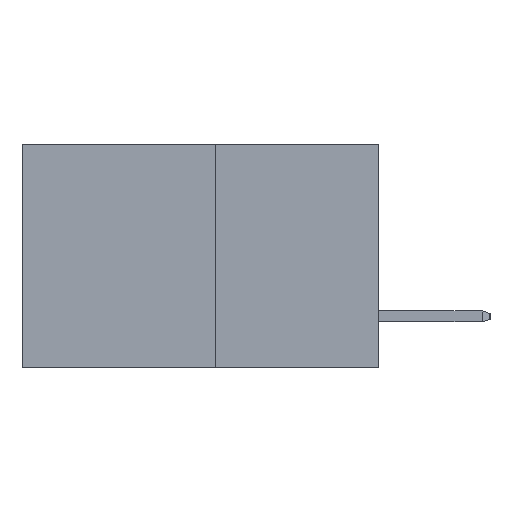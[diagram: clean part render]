
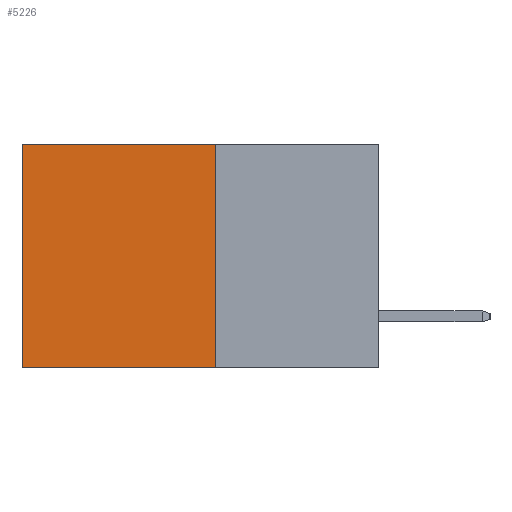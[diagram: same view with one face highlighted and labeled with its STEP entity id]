
A CAD part, left-side view. The second image highlights one B-rep face of the part: STEP entity #5226.
In plain terms, the highlighted planar face has unit normal (-1, 0, 0).
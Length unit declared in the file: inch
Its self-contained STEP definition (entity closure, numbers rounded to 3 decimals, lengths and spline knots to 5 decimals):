
#30 = PLANE ( 'NONE',  #6562 ) ;
#809 = VECTOR ( 'NONE', #12904, 39.37008 ) ;
#1406 = ORIENTED_EDGE ( 'NONE', *, *, #15030, .T. ) ;
#2121 = EDGE_LOOP ( 'NONE', ( #17578, #7805, #4749, #1406 ) ) ;
#4202 = CARTESIAN_POINT ( 'NONE',  ( 0.277, 0.27, 0. ) ) ;
#4749 = ORIENTED_EDGE ( 'NONE', *, *, #20772, .F. ) ;
#5063 = CARTESIAN_POINT ( 'NONE',  ( 0.277, 0.59, -0.37 ) ) ;
#5226 = ADVANCED_FACE ( 'NONE', ( #18118 ), #30, .F. ) ;
#5304 = LINE ( 'NONE', #11256, #809 ) ;
#6562 = AXIS2_PLACEMENT_3D ( 'NONE', #21273, #10420, #10381 ) ;
#7204 = CARTESIAN_POINT ( 'NONE',  ( 0.277, 0.59, 0. ) ) ;
#7753 = LINE ( 'NONE', #10885, #15904 ) ;
#7805 = ORIENTED_EDGE ( 'NONE', *, *, #10032, .F. ) ;
#7827 = EDGE_CURVE ( 'NONE', #16136, #9502, #19649, .T. ) ;
#8942 = LINE ( 'NONE', #4202, #13792 ) ;
#9502 = VERTEX_POINT ( 'NONE', #5063 ) ;
#10019 = CARTESIAN_POINT ( 'NONE',  ( 0.277, 0.27, -0.37 ) ) ;
#10032 = EDGE_CURVE ( 'NONE', #20286, #9502, #5304, .T. ) ;
#10381 = DIRECTION ( 'NONE',  ( 0., 0., -1. ) ) ;
#10420 = DIRECTION ( 'NONE',  ( 1., 0., 0. ) ) ;
#10885 = CARTESIAN_POINT ( 'NONE',  ( 0.277, 0.27, -0.37 ) ) ;
#11256 = CARTESIAN_POINT ( 'NONE',  ( 0.277, 0.27, -0.37 ) ) ;
#12085 = VECTOR ( 'NONE', #20454, 39.37008 ) ;
#12532 = DIRECTION ( 'NONE',  ( 0., 0., -1. ) ) ;
#12904 = DIRECTION ( 'NONE',  ( 0., 1., 0. ) ) ;
#13792 = VECTOR ( 'NONE', #18868, 39.37008 ) ;
#14789 = VERTEX_POINT ( 'NONE', #16710 ) ;
#15030 = EDGE_CURVE ( 'NONE', #14789, #16136, #8942, .T. ) ;
#15904 = VECTOR ( 'NONE', #12532, 39.37008 ) ;
#16136 = VERTEX_POINT ( 'NONE', #7204 ) ;
#16710 = CARTESIAN_POINT ( 'NONE',  ( 0.277, 0.27, 0. ) ) ;
#17578 = ORIENTED_EDGE ( 'NONE', *, *, #7827, .T. ) ;
#18118 = FACE_OUTER_BOUND ( 'NONE', #2121, .T. ) ;
#18868 = DIRECTION ( 'NONE',  ( 0., 1., 0. ) ) ;
#19649 = LINE ( 'NONE', #20539, #12085 ) ;
#20286 = VERTEX_POINT ( 'NONE', #10019 ) ;
#20454 = DIRECTION ( 'NONE',  ( 0., 0., -1. ) ) ;
#20539 = CARTESIAN_POINT ( 'NONE',  ( 0.277, 0.59, -0.37 ) ) ;
#20772 = EDGE_CURVE ( 'NONE', #14789, #20286, #7753, .T. ) ;
#21273 = CARTESIAN_POINT ( 'NONE',  ( 0.277, 0.27, -0.37 ) ) ;
